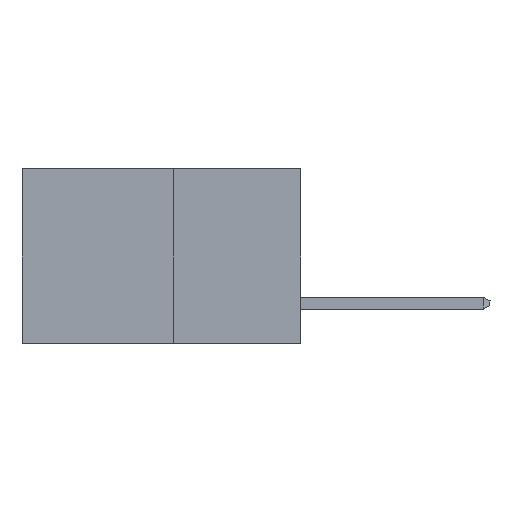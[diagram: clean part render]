
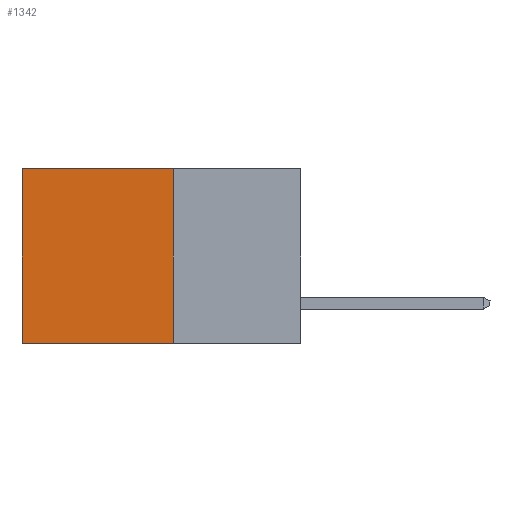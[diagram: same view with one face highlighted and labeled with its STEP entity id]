
A CAD part, left-side view. The second image highlights one B-rep face of the part: STEP entity #1342.
In plain terms, the highlighted planar face has unit normal (-1, 0, 0).
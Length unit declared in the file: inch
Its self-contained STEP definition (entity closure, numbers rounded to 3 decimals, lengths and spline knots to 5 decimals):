
#141 = CARTESIAN_POINT ( 'NONE',  ( 0.277, 0.27, -0.37 ) ) ;
#868 = EDGE_CURVE ( 'NONE', #5712, #3439, #6321, .T. ) ;
#1342 = ADVANCED_FACE ( 'NONE', ( #8880 ), #10484, .F. ) ;
#1668 = CARTESIAN_POINT ( 'NONE',  ( 0.277, 0.27, 0. ) ) ;
#2024 = VECTOR ( 'NONE', #3003, 39.37008 ) ;
#2193 = CARTESIAN_POINT ( 'NONE',  ( 0.277, 0.27, -0.37 ) ) ;
#2465 = VECTOR ( 'NONE', #8269, 39.37008 ) ;
#3003 = DIRECTION ( 'NONE',  ( 0., 0., -1. ) ) ;
#3345 = CARTESIAN_POINT ( 'NONE',  ( 0.277, 0.27, -0.37 ) ) ;
#3439 = VERTEX_POINT ( 'NONE', #3836 ) ;
#3836 = CARTESIAN_POINT ( 'NONE',  ( 0.277, 0.59, -0.37 ) ) ;
#4336 = EDGE_LOOP ( 'NONE', ( #5527, #10840, #13540, #5850 ) ) ;
#4734 = EDGE_CURVE ( 'NONE', #7338, #5712, #10562, .T. ) ;
#5527 = ORIENTED_EDGE ( 'NONE', *, *, #11911, .T. ) ;
#5712 = VERTEX_POINT ( 'NONE', #141 ) ;
#5850 = ORIENTED_EDGE ( 'NONE', *, *, #7248, .T. ) ;
#6068 = CARTESIAN_POINT ( 'NONE',  ( 0.277, 0.59, 0. ) ) ;
#6268 = CARTESIAN_POINT ( 'NONE',  ( 0.277, 0.27, 0. ) ) ;
#6321 = LINE ( 'NONE', #2193, #13648 ) ;
#7093 = VERTEX_POINT ( 'NONE', #6068 ) ;
#7131 = DIRECTION ( 'NONE',  ( 0., 1., 0. ) ) ;
#7248 = EDGE_CURVE ( 'NONE', #7338, #7093, #10898, .T. ) ;
#7338 = VERTEX_POINT ( 'NONE', #1668 ) ;
#7430 = VECTOR ( 'NONE', #9881, 39.37008 ) ;
#7878 = CARTESIAN_POINT ( 'NONE',  ( 0.277, 0.59, -0.37 ) ) ;
#8269 = DIRECTION ( 'NONE',  ( 0., 1., 0. ) ) ;
#8880 = FACE_OUTER_BOUND ( 'NONE', #4336, .T. ) ;
#9881 = DIRECTION ( 'NONE',  ( 0., 0., -1. ) ) ;
#10001 = AXIS2_PLACEMENT_3D ( 'NONE', #11649, #10481, #10273 ) ;
#10273 = DIRECTION ( 'NONE',  ( 0., 0., -1. ) ) ;
#10481 = DIRECTION ( 'NONE',  ( 1., 0., 0. ) ) ;
#10484 = PLANE ( 'NONE',  #10001 ) ;
#10562 = LINE ( 'NONE', #3345, #2024 ) ;
#10840 = ORIENTED_EDGE ( 'NONE', *, *, #868, .F. ) ;
#10898 = LINE ( 'NONE', #6268, #2465 ) ;
#11649 = CARTESIAN_POINT ( 'NONE',  ( 0.277, 0.27, -0.37 ) ) ;
#11911 = EDGE_CURVE ( 'NONE', #7093, #3439, #13052, .T. ) ;
#13052 = LINE ( 'NONE', #7878, #7430 ) ;
#13540 = ORIENTED_EDGE ( 'NONE', *, *, #4734, .F. ) ;
#13648 = VECTOR ( 'NONE', #7131, 39.37008 ) ;
